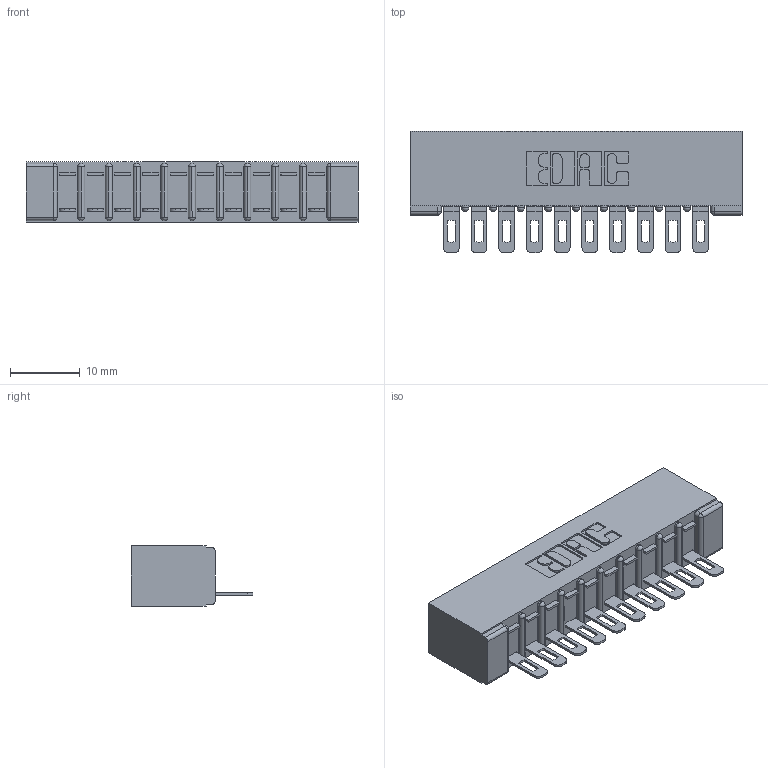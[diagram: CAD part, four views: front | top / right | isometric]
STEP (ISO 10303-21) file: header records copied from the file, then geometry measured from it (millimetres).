
FILE_DESCRIPTION (( 'STEP AP203' ), '1' );
FILE_NAME ('307-010-501-101.STEP', '2018-08-02T21:15:53', ( '' ), ( '' ), 'SwSTEP 2.0', 'SolidWorks 2016', '' );
FILE_SCHEMA (( 'CONFIG_CONTROL_DESIGN' ));
Length unit declared in the file: inch
Products named in the file (3): 307 Part_No Mounting Lugs; 307-290-002_501; 307-010-501-101
Assembly tree (11 placements, depth 2):
  307-010-501-101
    307 Part_No Mounting Lugs
    307-290-002_501  x10
Bounding box: 47.5 x 17.42 x 8.71 mm (x, y, z)
Volume: 3380.5 mm3; surface area: 6055.8 mm2
Topology: 11 solids, 11 shells, 881 faces, 2679 edges, 1754 vertices
Faces by surface type: plane 506, cylinder 353, sphere 22
Entity records: 13034 total; most frequent: CARTESIAN_POINT 2192, ORIENTED_EDGE 2182, DIRECTION 2147, EDGE_CURVE 1091, LINE 817, VECTOR 817, VERTEX_POINT 710, AXIS2_PLACEMENT_3D 665
